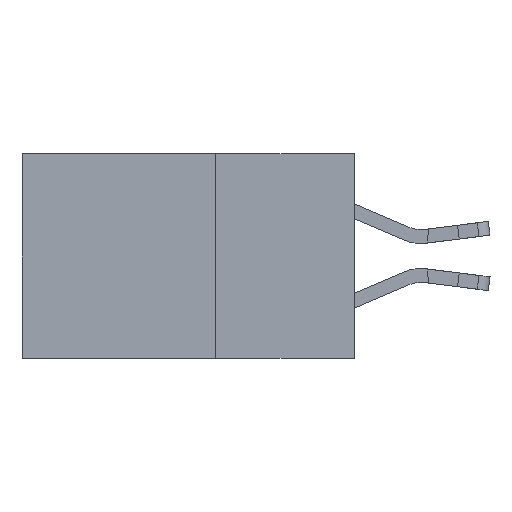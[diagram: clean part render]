
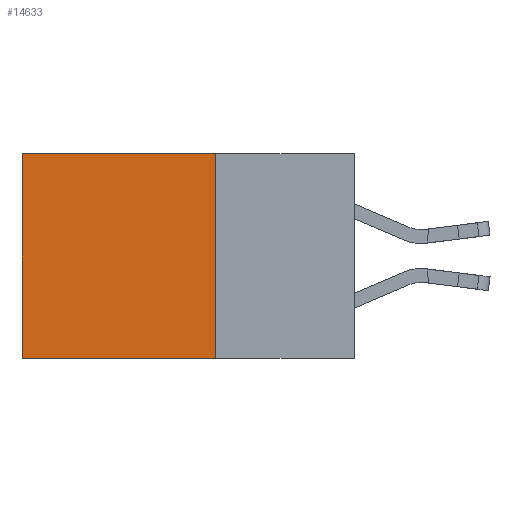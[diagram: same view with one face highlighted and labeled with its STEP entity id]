
A CAD part, left-side view. The second image highlights one B-rep face of the part: STEP entity #14633.
In plain terms, the highlighted planar face has unit normal (-1, 0, 0).
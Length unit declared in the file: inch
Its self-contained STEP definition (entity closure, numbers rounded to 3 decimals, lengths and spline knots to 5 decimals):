
#108 = ORIENTED_EDGE ( 'NONE', *, *, #10605, .T. ) ;
#345 = DIRECTION ( 'NONE',  ( 1., 0., 0. ) ) ;
#419 = FACE_OUTER_BOUND ( 'NONE', #3492, .T. ) ;
#751 = LINE ( 'NONE', #13501, #12671 ) ;
#1065 = EDGE_CURVE ( 'NONE', #2206, #4976, #3250, .T. ) ;
#2206 = VERTEX_POINT ( 'NONE', #7456 ) ;
#2617 = LINE ( 'NONE', #12399, #8866 ) ;
#3250 = LINE ( 'NONE', #12865, #6327 ) ;
#3492 = EDGE_LOOP ( 'NONE', ( #108, #13753, #11082, #5585 ) ) ;
#4037 = EDGE_CURVE ( 'NONE', #9880, #8622, #2617, .T. ) ;
#4976 = VERTEX_POINT ( 'NONE', #11837 ) ;
#5585 = ORIENTED_EDGE ( 'NONE', *, *, #1065, .T. ) ;
#5846 = CARTESIAN_POINT ( 'NONE',  ( 0.2615, 0.6, -0.37 ) ) ;
#6000 = AXIS2_PLACEMENT_3D ( 'NONE', #7354, #345, #8571 ) ;
#6094 = PLANE ( 'NONE',  #6000 ) ;
#6327 = VECTOR ( 'NONE', #12878, 39.37008 ) ;
#7352 = CARTESIAN_POINT ( 'NONE',  ( 0.2615, 0.25, -0.37 ) ) ;
#7354 = CARTESIAN_POINT ( 'NONE',  ( 0.2615, 0.25, -0.37 ) ) ;
#7456 = CARTESIAN_POINT ( 'NONE',  ( 0.2615, 0.25, 0. ) ) ;
#7707 = EDGE_CURVE ( 'NONE', #2206, #9880, #751, .T. ) ;
#8571 = DIRECTION ( 'NONE',  ( 0., 0., -1. ) ) ;
#8622 = VERTEX_POINT ( 'NONE', #5846 ) ;
#8866 = VECTOR ( 'NONE', #12366, 39.37008 ) ;
#9880 = VERTEX_POINT ( 'NONE', #7352 ) ;
#10272 = VECTOR ( 'NONE', #11260, 39.37008 ) ;
#10605 = EDGE_CURVE ( 'NONE', #4976, #8622, #10613, .T. ) ;
#10613 = LINE ( 'NONE', #14380, #10272 ) ;
#11082 = ORIENTED_EDGE ( 'NONE', *, *, #7707, .F. ) ;
#11260 = DIRECTION ( 'NONE',  ( 0., 0., -1. ) ) ;
#11837 = CARTESIAN_POINT ( 'NONE',  ( 0.2615, 0.6, 0. ) ) ;
#12366 = DIRECTION ( 'NONE',  ( 0., 1., 0. ) ) ;
#12399 = CARTESIAN_POINT ( 'NONE',  ( 0.2615, 0.25, -0.37 ) ) ;
#12671 = VECTOR ( 'NONE', #13518, 39.37008 ) ;
#12865 = CARTESIAN_POINT ( 'NONE',  ( 0.2615, 0.25, 0. ) ) ;
#12878 = DIRECTION ( 'NONE',  ( 0., 1., 0. ) ) ;
#13501 = CARTESIAN_POINT ( 'NONE',  ( 0.2615, 0.25, -0.37 ) ) ;
#13518 = DIRECTION ( 'NONE',  ( 0., 0., -1. ) ) ;
#13753 = ORIENTED_EDGE ( 'NONE', *, *, #4037, .F. ) ;
#14380 = CARTESIAN_POINT ( 'NONE',  ( 0.2615, 0.6, -0.37 ) ) ;
#14633 = ADVANCED_FACE ( 'NONE', ( #419 ), #6094, .F. ) ;
